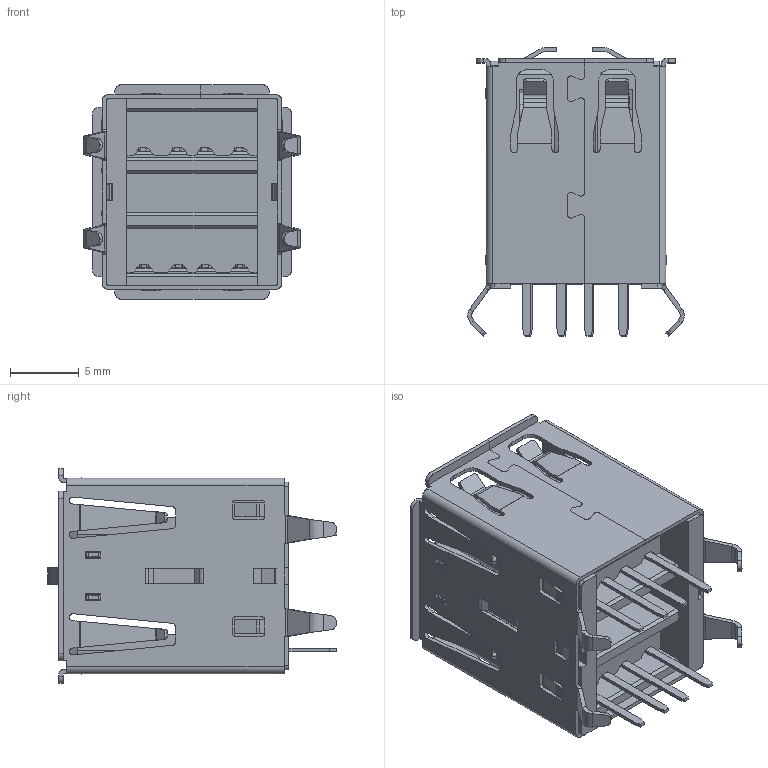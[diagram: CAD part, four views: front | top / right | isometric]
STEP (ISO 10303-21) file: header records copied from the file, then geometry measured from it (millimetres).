
FILE_DESCRIPTION (( 'STEP AP214' ), '1' );
FILE_NAME ('690N208-144-021.STEP', '2021-01-14T16:41:19', ( '' ), ( '' ), 'SwSTEP 2.0', 'SolidWorks 2020', '' );
FILE_SCHEMA (( 'AUTOMOTIVE_DESIGN' ));
Length unit declared in the file: millimetre
Products named in the file (14): Contact 7 690N208-X44-02X; Contact Lock Upper 690N208-X44-02X_Black; Contact 8 690N208-X44-02X; Insulator 690N208-X44-02X_Black; Contact 5 690N208-X44-02X; Contact 2 690N208-X44-02X; Contact 1 690N208-X44-02X; 690N208-144-021; Contact 4 690N208-X44-02X; Shell 2 690N208-X44-02X; Shell 690N208-X44-02X; Contact 3 690N208-X44-02X; Contact Lock Lower 690N208-X44-02X_Black; Contact 6 690N208-X44-02X
Assembly tree (13 placements, depth 2):
  690N208-144-021
    Shell 2 690N208-X44-02X
    Contact 6 690N208-X44-02X
    Contact 5 690N208-X44-02X
    Contact 7 690N208-X44-02X
    Contact 8 690N208-X44-02X
    Contact 2 690N208-X44-02X
    Contact 1 690N208-X44-02X
    Contact 3 690N208-X44-02X
    Contact 4 690N208-X44-02X
    Contact Lock Upper 690N208-X44-02X_Black
    Contact Lock Lower 690N208-X44-02X_Black
    Insulator 690N208-X44-02X_Black
    Shell 690N208-X44-02X
Bounding box: 15.78 x 21.02 x 15.64 mm (x, y, z)
Volume: 1797.2 mm3; surface area: 5239.8 mm2
Topology: 13 solids, 13 shells, 1538 faces, 4391 edges, 2863 vertices
Faces by surface type: plane 1164, cylinder 342, bspline 32
Entity records: 52276 total; most frequent: CARTESIAN_POINT 11925, ORIENTED_EDGE 8782, DIRECTION 7532, EDGE_CURVE 4391, LINE 3576, VECTOR 3576, VERTEX_POINT 2863, AXIS2_PLACEMENT_3D 1978
